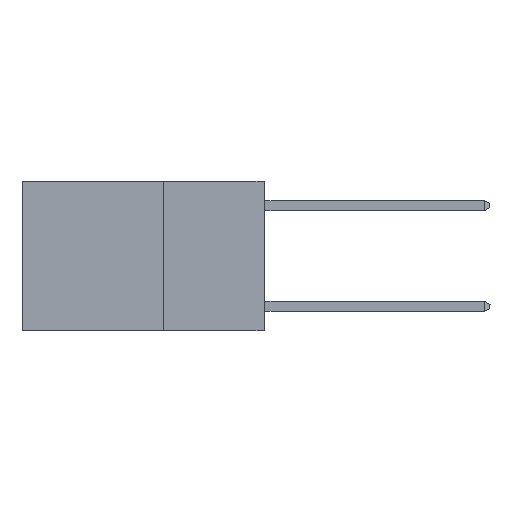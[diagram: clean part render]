
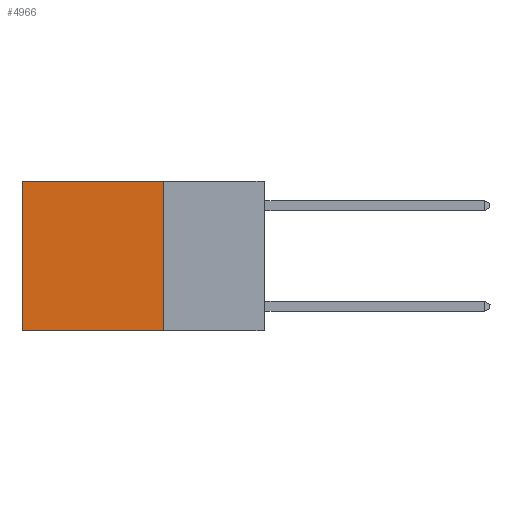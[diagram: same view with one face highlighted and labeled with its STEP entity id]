
A CAD part, left-side view. The second image highlights one B-rep face of the part: STEP entity #4966.
In plain terms, the highlighted planar face has unit normal (-1, 0, 0).
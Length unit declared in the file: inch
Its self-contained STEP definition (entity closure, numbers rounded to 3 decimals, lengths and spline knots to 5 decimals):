
#144 = DIRECTION ( 'NONE',  ( 1., 0., 0. ) ) ;
#852 = LINE ( 'NONE', #12355, #13400 ) ;
#1966 = CARTESIAN_POINT ( 'NONE',  ( 0.2625, 0.6, 0. ) ) ;
#2333 = EDGE_CURVE ( 'NONE', #2402, #19089, #852, .T. ) ;
#2402 = VERTEX_POINT ( 'NONE', #2640 ) ;
#2640 = CARTESIAN_POINT ( 'NONE',  ( 0.2625, 0.25, 0. ) ) ;
#3329 = CARTESIAN_POINT ( 'NONE',  ( 0.2625, 0.6, 0. ) ) ;
#4966 = ADVANCED_FACE ( 'NONE', ( #9566 ), #10065, .F. ) ;
#5057 = CARTESIAN_POINT ( 'NONE',  ( 0.2625, 0.25, 0. ) ) ;
#5114 = EDGE_LOOP ( 'NONE', ( #14582, #15072, #7147, #17091 ) ) ;
#7147 = ORIENTED_EDGE ( 'NONE', *, *, #14091, .F. ) ;
#7156 = VERTEX_POINT ( 'NONE', #20522 ) ;
#8508 = EDGE_CURVE ( 'NONE', #19089, #12126, #18838, .T. ) ;
#8800 = DIRECTION ( 'NONE',  ( 0., 1., 0. ) ) ;
#8999 = DIRECTION ( 'NONE',  ( 0., 1., 0. ) ) ;
#9566 = FACE_OUTER_BOUND ( 'NONE', #5114, .T. ) ;
#10065 = PLANE ( 'NONE',  #18684 ) ;
#10506 = CARTESIAN_POINT ( 'NONE',  ( 0.2625, 0.6, -0.37 ) ) ;
#11065 = VECTOR ( 'NONE', #14823, 39.37008 ) ;
#11681 = DIRECTION ( 'NONE',  ( 0., 0., -1. ) ) ;
#12126 = VERTEX_POINT ( 'NONE', #10506 ) ;
#12355 = CARTESIAN_POINT ( 'NONE',  ( 0.2625, 0.25, 0. ) ) ;
#12778 = LINE ( 'NONE', #16833, #20607 ) ;
#13400 = VECTOR ( 'NONE', #8999, 39.37008 ) ;
#14091 = EDGE_CURVE ( 'NONE', #2402, #7156, #19921, .T. ) ;
#14582 = ORIENTED_EDGE ( 'NONE', *, *, #8508, .T. ) ;
#14677 = VECTOR ( 'NONE', #14988, 39.37008 ) ;
#14823 = DIRECTION ( 'NONE',  ( 0., 0., -1. ) ) ;
#14988 = DIRECTION ( 'NONE',  ( 0., 0., -1. ) ) ;
#15072 = ORIENTED_EDGE ( 'NONE', *, *, #15647, .F. ) ;
#15647 = EDGE_CURVE ( 'NONE', #7156, #12126, #12778, .T. ) ;
#16833 = CARTESIAN_POINT ( 'NONE',  ( 0.2625, 0.25, -0.37 ) ) ;
#17091 = ORIENTED_EDGE ( 'NONE', *, *, #2333, .T. ) ;
#18684 = AXIS2_PLACEMENT_3D ( 'NONE', #19507, #144, #11681 ) ;
#18838 = LINE ( 'NONE', #1966, #14677 ) ;
#19089 = VERTEX_POINT ( 'NONE', #3329 ) ;
#19507 = CARTESIAN_POINT ( 'NONE',  ( 0.2625, 0.25, 0. ) ) ;
#19921 = LINE ( 'NONE', #5057, #11065 ) ;
#20522 = CARTESIAN_POINT ( 'NONE',  ( 0.2625, 0.25, -0.37 ) ) ;
#20607 = VECTOR ( 'NONE', #8800, 39.37008 ) ;
